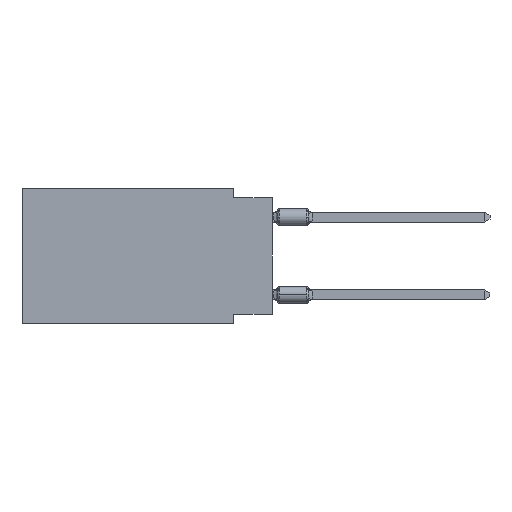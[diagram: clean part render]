
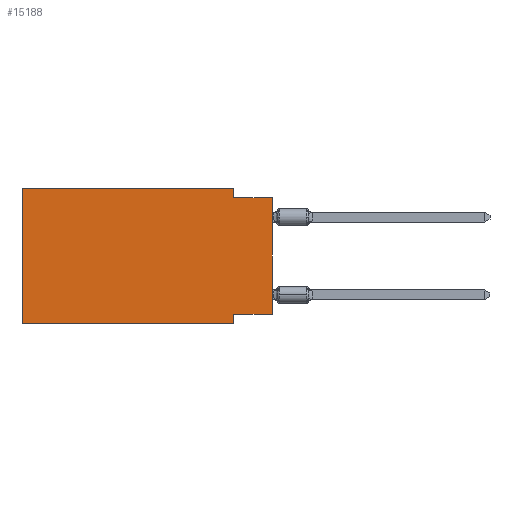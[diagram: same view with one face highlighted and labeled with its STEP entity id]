
A CAD part, left-side view. The second image highlights one B-rep face of the part: STEP entity #15188.
In plain terms, the highlighted planar face has unit normal (-1, 0, 0).
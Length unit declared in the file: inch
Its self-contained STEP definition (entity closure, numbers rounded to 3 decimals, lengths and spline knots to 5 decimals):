
#1130 = LINE ( 'NONE', #14751, #11804 ) ;
#1344 = LINE ( 'NONE', #7383, #2988 ) ;
#1373 = VECTOR ( 'NONE', #22396, 39.37008 ) ;
#1475 = CARTESIAN_POINT ( 'NONE',  ( 0., 0., -0.025 ) ) ;
#1713 = ORIENTED_EDGE ( 'NONE', *, *, #20534, .F. ) ;
#1851 = ORIENTED_EDGE ( 'NONE', *, *, #9595, .T. ) ;
#2330 = LINE ( 'NONE', #16307, #17294 ) ;
#2376 = CARTESIAN_POINT ( 'NONE',  ( 0., 0., -0.325 ) ) ;
#2614 = VECTOR ( 'NONE', #12115, 39.37008 ) ;
#2988 = VECTOR ( 'NONE', #23332, 39.37008 ) ;
#4014 = VERTEX_POINT ( 'NONE', #17319 ) ;
#4578 = CARTESIAN_POINT ( 'NONE',  ( 0., 0.645, 0. ) ) ;
#4824 = DIRECTION ( 'NONE',  ( 0., -1., 0. ) ) ;
#4926 = CARTESIAN_POINT ( 'NONE',  ( 0., 0.645, -0.35 ) ) ;
#5048 = CARTESIAN_POINT ( 'NONE',  ( 0., 0., 0. ) ) ;
#5905 = EDGE_CURVE ( 'NONE', #18496, #17172, #1130, .T. ) ;
#6204 = FACE_OUTER_BOUND ( 'NONE', #17080, .T. ) ;
#6267 = VECTOR ( 'NONE', #18592, 39.37008 ) ;
#7383 = CARTESIAN_POINT ( 'NONE',  ( 0., 0.1, 0. ) ) ;
#8388 = ORIENTED_EDGE ( 'NONE', *, *, #25234, .F. ) ;
#8624 = CARTESIAN_POINT ( 'NONE',  ( 0., 0.1, -0.025 ) ) ;
#8661 = EDGE_CURVE ( 'NONE', #22558, #12101, #11997, .T. ) ;
#9595 = EDGE_CURVE ( 'NONE', #4014, #15408, #22981, .T. ) ;
#10072 = ORIENTED_EDGE ( 'NONE', *, *, #10207, .F. ) ;
#10207 = EDGE_CURVE ( 'NONE', #19244, #15041, #1344, .T. ) ;
#10988 = ORIENTED_EDGE ( 'NONE', *, *, #8661, .F. ) ;
#11096 = AXIS2_PLACEMENT_3D ( 'NONE', #14179, #12227, #20338 ) ;
#11210 = EDGE_CURVE ( 'NONE', #18496, #12101, #2330, .T. ) ;
#11804 = VECTOR ( 'NONE', #12918, 39.37008 ) ;
#11997 = LINE ( 'NONE', #19972, #2614 ) ;
#12101 = VERTEX_POINT ( 'NONE', #19491 ) ;
#12115 = DIRECTION ( 'NONE',  ( 0., 0., -1. ) ) ;
#12227 = DIRECTION ( 'NONE',  ( 1., 0., 0. ) ) ;
#12418 = LINE ( 'NONE', #22360, #14628 ) ;
#12918 = DIRECTION ( 'NONE',  ( 0., 0., 1. ) ) ;
#13851 = CARTESIAN_POINT ( 'NONE',  ( 0., 0.1, 0. ) ) ;
#14066 = PLANE ( 'NONE',  #11096 ) ;
#14179 = CARTESIAN_POINT ( 'NONE',  ( 0., 0.645, 0. ) ) ;
#14628 = VECTOR ( 'NONE', #4824, 39.37008 ) ;
#14751 = CARTESIAN_POINT ( 'NONE',  ( 0., 0.645, 0. ) ) ;
#14788 = VECTOR ( 'NONE', #20898, 39.37008 ) ;
#15041 = VERTEX_POINT ( 'NONE', #8624 ) ;
#15188 = ADVANCED_FACE ( 'NONE', ( #6204 ), #14066, .F. ) ;
#15408 = VERTEX_POINT ( 'NONE', #1475 ) ;
#16307 = CARTESIAN_POINT ( 'NONE',  ( 0., 0.645, -0.35 ) ) ;
#16401 = ORIENTED_EDGE ( 'NONE', *, *, #11210, .T. ) ;
#17080 = EDGE_LOOP ( 'NONE', ( #1851, #1713, #10072, #24614, #18732, #16401, #10988, #8388 ) ) ;
#17172 = VERTEX_POINT ( 'NONE', #24057 ) ;
#17294 = VECTOR ( 'NONE', #18551, 39.37008 ) ;
#17319 = CARTESIAN_POINT ( 'NONE',  ( 0., 0., -0.325 ) ) ;
#18330 = LINE ( 'NONE', #2376, #1373 ) ;
#18496 = VERTEX_POINT ( 'NONE', #4926 ) ;
#18551 = DIRECTION ( 'NONE',  ( 0., -1., 0. ) ) ;
#18592 = DIRECTION ( 'NONE',  ( 0., -1., 0. ) ) ;
#18732 = ORIENTED_EDGE ( 'NONE', *, *, #5905, .F. ) ;
#19244 = VERTEX_POINT ( 'NONE', #13851 ) ;
#19491 = CARTESIAN_POINT ( 'NONE',  ( 0., 0.1, -0.35 ) ) ;
#19972 = CARTESIAN_POINT ( 'NONE',  ( 0., 0.1, -0.35 ) ) ;
#20064 = EDGE_CURVE ( 'NONE', #17172, #19244, #22784, .T. ) ;
#20338 = DIRECTION ( 'NONE',  ( 0., 0., -1. ) ) ;
#20534 = EDGE_CURVE ( 'NONE', #15041, #15408, #12418, .T. ) ;
#20898 = DIRECTION ( 'NONE',  ( 0., 0., 1. ) ) ;
#22360 = CARTESIAN_POINT ( 'NONE',  ( 0., 0., -0.025 ) ) ;
#22396 = DIRECTION ( 'NONE',  ( 0., 1., 0. ) ) ;
#22558 = VERTEX_POINT ( 'NONE', #25577 ) ;
#22784 = LINE ( 'NONE', #4578, #6267 ) ;
#22981 = LINE ( 'NONE', #5048, #14788 ) ;
#23332 = DIRECTION ( 'NONE',  ( 0., 0., -1. ) ) ;
#24057 = CARTESIAN_POINT ( 'NONE',  ( 0., 0.645, 0. ) ) ;
#24614 = ORIENTED_EDGE ( 'NONE', *, *, #20064, .F. ) ;
#25234 = EDGE_CURVE ( 'NONE', #4014, #22558, #18330, .T. ) ;
#25577 = CARTESIAN_POINT ( 'NONE',  ( 0., 0.1, -0.325 ) ) ;
